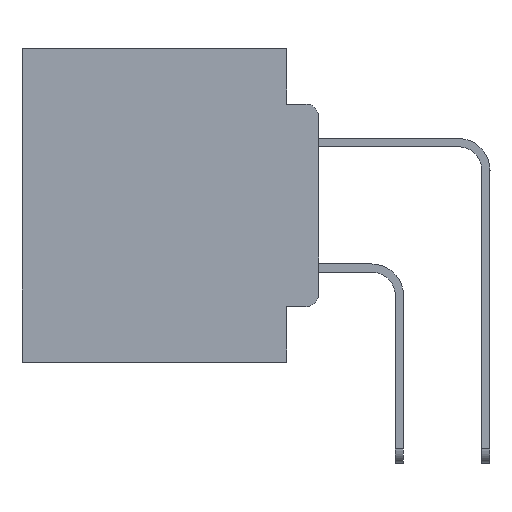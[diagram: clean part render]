
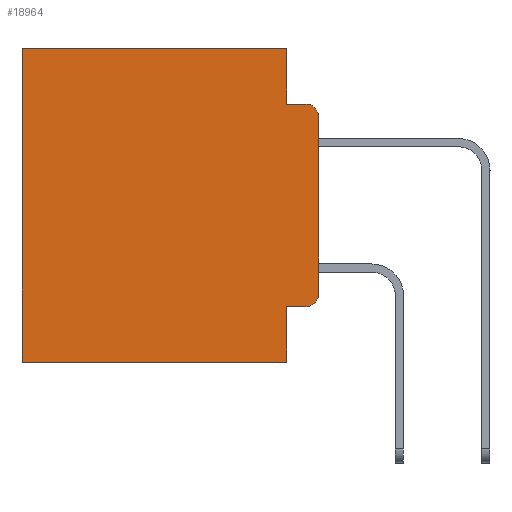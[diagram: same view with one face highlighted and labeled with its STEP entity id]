
A CAD part, left-side view. The second image highlights one B-rep face of the part: STEP entity #18964.
In plain terms, the highlighted planar face has unit normal (-1, 0, 0).
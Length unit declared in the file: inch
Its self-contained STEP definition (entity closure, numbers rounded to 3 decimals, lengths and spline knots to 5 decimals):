
#321 = CARTESIAN_POINT ( 'NONE',  ( 0.298, 0., -0.3915 ) ) ;
#421 = ORIENTED_EDGE ( 'NONE', *, *, #23379, .T. ) ;
#1428 = EDGE_CURVE ( 'NONE', #6171, #1645, #7738, .T. ) ;
#1558 = CARTESIAN_POINT ( 'NONE',  ( 0.298, 0.051, -0.0885 ) ) ;
#1645 = VERTEX_POINT ( 'NONE', #321 ) ;
#1738 = VECTOR ( 'NONE', #10694, 39.37008 ) ;
#1982 = CARTESIAN_POINT ( 'NONE',  ( 0.298, 0., 0. ) ) ;
#2089 = CARTESIAN_POINT ( 'NONE',  ( 0.298, 0.02, -0.3915 ) ) ;
#2625 = ORIENTED_EDGE ( 'NONE', *, *, #28575, .T. ) ;
#2901 = EDGE_CURVE ( 'NONE', #7442, #15600, #19163, .T. ) ;
#3280 = DIRECTION ( 'NONE',  ( 1., 0., 0. ) ) ;
#3372 = PLANE ( 'NONE',  #21264 ) ;
#3787 = CARTESIAN_POINT ( 'NONE',  ( 0.298, 0.051, 0. ) ) ;
#4503 = VERTEX_POINT ( 'NONE', #1558 ) ;
#4810 = FACE_OUTER_BOUND ( 'NONE', #29606, .T. ) ;
#5066 = CARTESIAN_POINT ( 'NONE',  ( 0.298, 0., -0.5 ) ) ;
#5198 = CARTESIAN_POINT ( 'NONE',  ( 0.298, 0.051, -0.4115 ) ) ;
#5422 = CIRCLE ( 'NONE', #22267, 0.02 ) ;
#5825 = CARTESIAN_POINT ( 'NONE',  ( 0.298, 0.02, -0.1085 ) ) ;
#6171 = VERTEX_POINT ( 'NONE', #30778 ) ;
#6184 = DIRECTION ( 'NONE',  ( 0., 0., -1. ) ) ;
#6473 = AXIS2_PLACEMENT_3D ( 'NONE', #2089, #20918, #23767 ) ;
#7204 = DIRECTION ( 'NONE',  ( 0., 1., 0. ) ) ;
#7305 = VERTEX_POINT ( 'NONE', #14987 ) ;
#7442 = VERTEX_POINT ( 'NONE', #15481 ) ;
#7738 = CIRCLE ( 'NONE', #6473, 0.02 ) ;
#8147 = CARTESIAN_POINT ( 'NONE',  ( 0.298, 0.051, 0. ) ) ;
#8232 = DIRECTION ( 'NONE',  ( 0., 0., -1. ) ) ;
#8273 = ORIENTED_EDGE ( 'NONE', *, *, #28438, .F. ) ;
#8671 = VERTEX_POINT ( 'NONE', #11296 ) ;
#8839 = VECTOR ( 'NONE', #17032, 39.37008 ) ;
#9479 = LINE ( 'NONE', #1982, #9519 ) ;
#9519 = VECTOR ( 'NONE', #25947, 39.37008 ) ;
#10518 = DIRECTION ( 'NONE',  ( 0., 0., -1. ) ) ;
#10694 = DIRECTION ( 'NONE',  ( 0., -1., 0. ) ) ;
#10853 = VECTOR ( 'NONE', #7204, 39.37008 ) ;
#11296 = CARTESIAN_POINT ( 'NONE',  ( 0.298, 0., -0.1085 ) ) ;
#11982 = ORIENTED_EDGE ( 'NONE', *, *, #29997, .T. ) ;
#12079 = VECTOR ( 'NONE', #10518, 39.37008 ) ;
#12117 = ORIENTED_EDGE ( 'NONE', *, *, #2901, .F. ) ;
#12839 = VECTOR ( 'NONE', #24262, 39.37008 ) ;
#13201 = CARTESIAN_POINT ( 'NONE',  ( 0.298, 0.051, -0.4115 ) ) ;
#13396 = ORIENTED_EDGE ( 'NONE', *, *, #21266, .F. ) ;
#13519 = LINE ( 'NONE', #13201, #21330 ) ;
#13545 = CARTESIAN_POINT ( 'NONE',  ( 0.298, 0.051, 0. ) ) ;
#14987 = CARTESIAN_POINT ( 'NONE',  ( 0.298, 0.473, 0. ) ) ;
#15460 = DIRECTION ( 'NONE',  ( 0., 0., -1. ) ) ;
#15481 = CARTESIAN_POINT ( 'NONE',  ( 0.298, 0.051, -0.5 ) ) ;
#15600 = VERTEX_POINT ( 'NONE', #29177 ) ;
#15904 = LINE ( 'NONE', #20089, #1738 ) ;
#17032 = DIRECTION ( 'NONE',  ( 0., 0., -1. ) ) ;
#17733 = CARTESIAN_POINT ( 'NONE',  ( 0.298, 0., 0. ) ) ;
#17867 = ORIENTED_EDGE ( 'NONE', *, *, #26843, .F. ) ;
#17937 = EDGE_CURVE ( 'NONE', #4503, #29288, #15904, .T. ) ;
#18012 = DIRECTION ( 'NONE',  ( -1., 0., 0. ) ) ;
#18964 = ADVANCED_FACE ( 'NONE', ( #4810 ), #3372, .F. ) ;
#19163 = LINE ( 'NONE', #5066, #12839 ) ;
#19235 = CARTESIAN_POINT ( 'NONE',  ( 0.298, 0.02, -0.0885 ) ) ;
#19806 = VERTEX_POINT ( 'NONE', #13545 ) ;
#20089 = CARTESIAN_POINT ( 'NONE',  ( 0.298, 0.051, -0.0885 ) ) ;
#20918 = DIRECTION ( 'NONE',  ( -1., 0., 0. ) ) ;
#20955 = VECTOR ( 'NONE', #6184, 39.37008 ) ;
#21264 = AXIS2_PLACEMENT_3D ( 'NONE', #17733, #3280, #15460 ) ;
#21266 = EDGE_CURVE ( 'NONE', #8671, #1645, #9479, .T. ) ;
#21330 = VECTOR ( 'NONE', #29879, 39.37008 ) ;
#22267 = AXIS2_PLACEMENT_3D ( 'NONE', #5825, #18012, #8232 ) ;
#23379 = EDGE_CURVE ( 'NONE', #24153, #6171, #13519, .T. ) ;
#23767 = DIRECTION ( 'NONE',  ( 0., 0., -1. ) ) ;
#23882 = ORIENTED_EDGE ( 'NONE', *, *, #17937, .F. ) ;
#24146 = ORIENTED_EDGE ( 'NONE', *, *, #1428, .T. ) ;
#24153 = VERTEX_POINT ( 'NONE', #5198 ) ;
#24262 = DIRECTION ( 'NONE',  ( 0., 1., 0. ) ) ;
#24336 = LINE ( 'NONE', #3787, #20955 ) ;
#25947 = DIRECTION ( 'NONE',  ( 0., 0., -1. ) ) ;
#26506 = CARTESIAN_POINT ( 'NONE',  ( 0.298, 0.473, 0. ) ) ;
#26559 = LINE ( 'NONE', #28885, #10853 ) ;
#26615 = LINE ( 'NONE', #8147, #12079 ) ;
#26843 = EDGE_CURVE ( 'NONE', #19806, #4503, #26615, .T. ) ;
#27853 = LINE ( 'NONE', #26506, #8839 ) ;
#28438 = EDGE_CURVE ( 'NONE', #24153, #7442, #24336, .T. ) ;
#28575 = EDGE_CURVE ( 'NONE', #19806, #7305, #26559, .T. ) ;
#28885 = CARTESIAN_POINT ( 'NONE',  ( 0.298, 0., 0. ) ) ;
#29177 = CARTESIAN_POINT ( 'NONE',  ( 0.298, 0.473, -0.5 ) ) ;
#29288 = VERTEX_POINT ( 'NONE', #19235 ) ;
#29326 = ORIENTED_EDGE ( 'NONE', *, *, #30759, .T. ) ;
#29606 = EDGE_LOOP ( 'NONE', ( #13396, #29326, #23882, #17867, #2625, #11982, #12117, #8273, #421, #24146 ) ) ;
#29879 = DIRECTION ( 'NONE',  ( 0., -1., 0. ) ) ;
#29997 = EDGE_CURVE ( 'NONE', #7305, #15600, #27853, .T. ) ;
#30759 = EDGE_CURVE ( 'NONE', #8671, #29288, #5422, .T. ) ;
#30778 = CARTESIAN_POINT ( 'NONE',  ( 0.298, 0.02, -0.4115 ) ) ;
